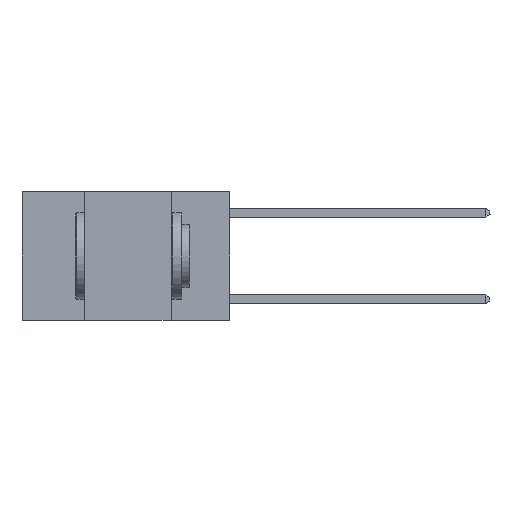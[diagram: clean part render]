
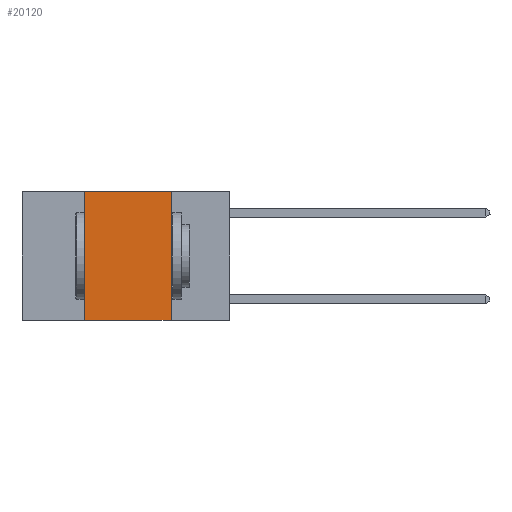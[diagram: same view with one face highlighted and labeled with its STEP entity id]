
A CAD part, left-side view. The second image highlights one B-rep face of the part: STEP entity #20120.
In plain terms, the highlighted planar face has unit normal (-1, 0, 0).
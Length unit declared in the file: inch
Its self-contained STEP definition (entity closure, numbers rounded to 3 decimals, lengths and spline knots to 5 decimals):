
#58 = DIRECTION ( 'NONE',  ( 0., -1., 0. ) ) ;
#568 = EDGE_CURVE ( 'NONE', #2918, #16182, #20295, .T. ) ;
#1155 = AXIS2_PLACEMENT_3D ( 'NONE', #21616, #7005, #1634 ) ;
#1634 = DIRECTION ( 'NONE',  ( 0., 0., -1. ) ) ;
#1967 = CARTESIAN_POINT ( 'NONE',  ( 0., 0.6, 0. ) ) ;
#2025 = EDGE_CURVE ( 'NONE', #16182, #13966, #14799, .T. ) ;
#2760 = ORIENTED_EDGE ( 'NONE', *, *, #16031, .T. ) ;
#2918 = VERTEX_POINT ( 'NONE', #5786 ) ;
#3078 = EDGE_LOOP ( 'NONE', ( #17714, #15230, #22892, #2760 ) ) ;
#4053 = VECTOR ( 'NONE', #14326, 39.37008 ) ;
#5186 = DIRECTION ( 'NONE',  ( 0., -1., 0. ) ) ;
#5331 = VECTOR ( 'NONE', #5186, 39.37008 ) ;
#5469 = LINE ( 'NONE', #8778, #19800 ) ;
#5786 = CARTESIAN_POINT ( 'NONE',  ( 0., 0.42, -0.37 ) ) ;
#5793 = CARTESIAN_POINT ( 'NONE',  ( 0., 0.17, -0.37 ) ) ;
#6212 = VECTOR ( 'NONE', #58, 39.37008 ) ;
#6565 = CARTESIAN_POINT ( 'NONE',  ( 0., 0.17, 0. ) ) ;
#7005 = DIRECTION ( 'NONE',  ( 1., 0., 0. ) ) ;
#8778 = CARTESIAN_POINT ( 'NONE',  ( 0., 0.17, 0. ) ) ;
#10675 = FACE_OUTER_BOUND ( 'NONE', #3078, .T. ) ;
#13355 = CARTESIAN_POINT ( 'NONE',  ( 0., 0.42, 0. ) ) ;
#13966 = VERTEX_POINT ( 'NONE', #6565 ) ;
#14326 = DIRECTION ( 'NONE',  ( 0., 0., 1. ) ) ;
#14436 = CARTESIAN_POINT ( 'NONE',  ( 0., 0.6, -0.37 ) ) ;
#14799 = LINE ( 'NONE', #1967, #6212 ) ;
#15185 = VERTEX_POINT ( 'NONE', #5793 ) ;
#15230 = ORIENTED_EDGE ( 'NONE', *, *, #2025, .F. ) ;
#16031 = EDGE_CURVE ( 'NONE', #2918, #15185, #19941, .T. ) ;
#16182 = VERTEX_POINT ( 'NONE', #13355 ) ;
#17714 = ORIENTED_EDGE ( 'NONE', *, *, #20091, .F. ) ;
#18179 = DIRECTION ( 'NONE',  ( 0., 0., -1. ) ) ;
#19800 = VECTOR ( 'NONE', #18179, 39.37008 ) ;
#19941 = LINE ( 'NONE', #14436, #5331 ) ;
#20055 = CARTESIAN_POINT ( 'NONE',  ( 0., 0.42, 0. ) ) ;
#20091 = EDGE_CURVE ( 'NONE', #13966, #15185, #5469, .T. ) ;
#20120 = ADVANCED_FACE ( 'NONE', ( #10675 ), #21394, .F. ) ;
#20295 = LINE ( 'NONE', #20055, #4053 ) ;
#21394 = PLANE ( 'NONE',  #1155 ) ;
#21616 = CARTESIAN_POINT ( 'NONE',  ( 0., 0.6, 0. ) ) ;
#22892 = ORIENTED_EDGE ( 'NONE', *, *, #568, .F. ) ;
